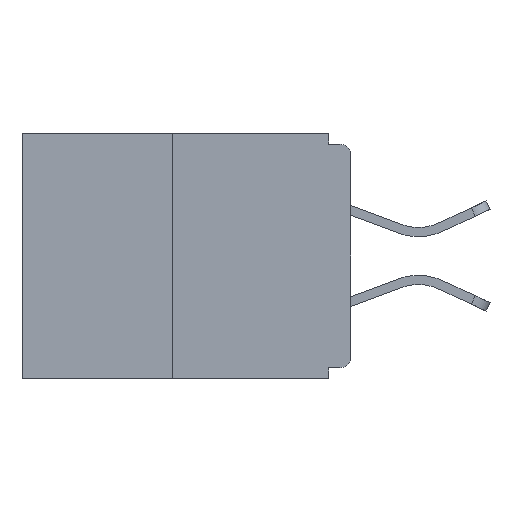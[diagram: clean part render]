
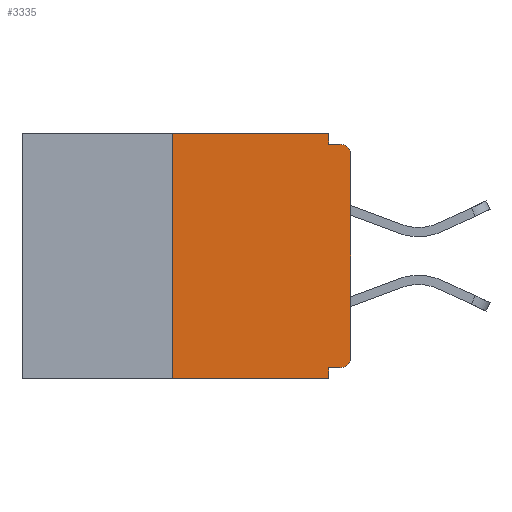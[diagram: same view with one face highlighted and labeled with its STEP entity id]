
A CAD part, left-side view. The second image highlights one B-rep face of the part: STEP entity #3335.
In plain terms, the highlighted planar face has unit normal (-1, 0, 0).
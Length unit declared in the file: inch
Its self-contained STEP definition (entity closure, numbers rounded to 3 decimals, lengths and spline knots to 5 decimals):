
#395 = EDGE_CURVE ( 'NONE', #3561, #10887, #11701, .T. ) ;
#424 = ORIENTED_EDGE ( 'NONE', *, *, #395, .F. ) ;
#631 = AXIS2_PLACEMENT_3D ( 'NONE', #7756, #4073, #10716 ) ;
#733 = AXIS2_PLACEMENT_3D ( 'NONE', #6651, #11321, #5610 ) ;
#974 = EDGE_CURVE ( 'NONE', #9422, #10626, #7133, .T. ) ;
#1036 = CARTESIAN_POINT ( 'NONE',  ( 0., 0.031, -0.015 ) ) ;
#1272 = LINE ( 'NONE', #4198, #9743 ) ;
#1452 = DIRECTION ( 'NONE',  ( 0., 0., 1. ) ) ;
#1589 = DIRECTION ( 'NONE',  ( -1., 0., 0. ) ) ;
#1690 = CARTESIAN_POINT ( 'NONE',  ( 0., 0.015, -0.313 ) ) ;
#2043 = DIRECTION ( 'NONE',  ( 0., -1., 0. ) ) ;
#2062 = ORIENTED_EDGE ( 'NONE', *, *, #2302, .F. ) ;
#2302 = EDGE_CURVE ( 'NONE', #11310, #5350, #6602, .T. ) ;
#2515 = CARTESIAN_POINT ( 'NONE',  ( 0., 0.015, -0.015 ) ) ;
#2636 = CARTESIAN_POINT ( 'NONE',  ( 0., 0.015, -0.328 ) ) ;
#2792 = VECTOR ( 'NONE', #6724, 39.37008 ) ;
#2806 = ORIENTED_EDGE ( 'NONE', *, *, #4476, .T. ) ;
#3335 = ADVANCED_FACE ( 'NONE', ( #8786 ), #8521, .F. ) ;
#3561 = VERTEX_POINT ( 'NONE', #5528 ) ;
#3802 = CARTESIAN_POINT ( 'NONE',  ( 0., 0., -0.03 ) ) ;
#3863 = CARTESIAN_POINT ( 'NONE',  ( 0., 0., -0.328 ) ) ;
#4073 = DIRECTION ( 'NONE',  ( -1., 0., 0. ) ) ;
#4198 = CARTESIAN_POINT ( 'NONE',  ( 0., 0.25, 0. ) ) ;
#4236 = VECTOR ( 'NONE', #1452, 39.37008 ) ;
#4357 = CARTESIAN_POINT ( 'NONE',  ( 0., 0.031, -0.343 ) ) ;
#4476 = EDGE_CURVE ( 'NONE', #5904, #5350, #11220, .T. ) ;
#4690 = LINE ( 'NONE', #7128, #4236 ) ;
#4773 = ORIENTED_EDGE ( 'NONE', *, *, #9515, .F. ) ;
#4829 = VECTOR ( 'NONE', #5130, 39.37008 ) ;
#4846 = CARTESIAN_POINT ( 'NONE',  ( 0., 0., -0.313 ) ) ;
#4853 = EDGE_CURVE ( 'NONE', #8885, #10826, #8806, .T. ) ;
#4958 = DIRECTION ( 'NONE',  ( 0., 0., 1. ) ) ;
#5130 = DIRECTION ( 'NONE',  ( 0., 0., -1. ) ) ;
#5167 = EDGE_CURVE ( 'NONE', #10887, #10626, #6867, .T. ) ;
#5242 = VECTOR ( 'NONE', #2043, 39.37008 ) ;
#5350 = VERTEX_POINT ( 'NONE', #4357 ) ;
#5528 = CARTESIAN_POINT ( 'NONE',  ( 0., 0.031, 0. ) ) ;
#5610 = DIRECTION ( 'NONE',  ( 0., 0., -1. ) ) ;
#5904 = VERTEX_POINT ( 'NONE', #11522 ) ;
#6077 = ORIENTED_EDGE ( 'NONE', *, *, #9986, .T. ) ;
#6602 = LINE ( 'NONE', #10877, #4829 ) ;
#6651 = CARTESIAN_POINT ( 'NONE',  ( 0., 0.46, 0. ) ) ;
#6724 = DIRECTION ( 'NONE',  ( 0., 0., -1. ) ) ;
#6867 = LINE ( 'NONE', #7733, #5242 ) ;
#7065 = EDGE_LOOP ( 'NONE', ( #8903, #10130, #2806, #2062, #4773, #9721, #6077, #9831, #12045, #424 ) ) ;
#7128 = CARTESIAN_POINT ( 'NONE',  ( 0., 0., 0. ) ) ;
#7133 = CIRCLE ( 'NONE', #631, 0.015 ) ;
#7208 = DIRECTION ( 'NONE',  ( 0., 0., -1. ) ) ;
#7671 = CARTESIAN_POINT ( 'NONE',  ( 0., 0.031, 0. ) ) ;
#7733 = CARTESIAN_POINT ( 'NONE',  ( 0., 0., -0.015 ) ) ;
#7756 = CARTESIAN_POINT ( 'NONE',  ( 0., 0.015, -0.03 ) ) ;
#7925 = VECTOR ( 'NONE', #12298, 39.37008 ) ;
#8292 = CARTESIAN_POINT ( 'NONE',  ( 0., 0.46, 0. ) ) ;
#8434 = DIRECTION ( 'NONE',  ( 0., 1., 0. ) ) ;
#8521 = PLANE ( 'NONE',  #733 ) ;
#8569 = EDGE_CURVE ( 'NONE', #9332, #3561, #10972, .T. ) ;
#8661 = DIRECTION ( 'NONE',  ( 0., -1., 0. ) ) ;
#8786 = FACE_OUTER_BOUND ( 'NONE', #7065, .T. ) ;
#8806 = CIRCLE ( 'NONE', #9650, 0.015 ) ;
#8885 = VERTEX_POINT ( 'NONE', #2636 ) ;
#8903 = ORIENTED_EDGE ( 'NONE', *, *, #8569, .F. ) ;
#9139 = CARTESIAN_POINT ( 'NONE',  ( 0., 0.031, -0.328 ) ) ;
#9315 = VECTOR ( 'NONE', #8661, 39.37008 ) ;
#9332 = VERTEX_POINT ( 'NONE', #11572 ) ;
#9422 = VERTEX_POINT ( 'NONE', #3802 ) ;
#9515 = EDGE_CURVE ( 'NONE', #8885, #11310, #10366, .T. ) ;
#9650 = AXIS2_PLACEMENT_3D ( 'NONE', #1690, #1589, #7208 ) ;
#9721 = ORIENTED_EDGE ( 'NONE', *, *, #4853, .T. ) ;
#9743 = VECTOR ( 'NONE', #4958, 39.37008 ) ;
#9823 = EDGE_CURVE ( 'NONE', #5904, #9332, #1272, .T. ) ;
#9831 = ORIENTED_EDGE ( 'NONE', *, *, #974, .T. ) ;
#9986 = EDGE_CURVE ( 'NONE', #10826, #9422, #4690, .T. ) ;
#10130 = ORIENTED_EDGE ( 'NONE', *, *, #9823, .F. ) ;
#10366 = LINE ( 'NONE', #3863, #10512 ) ;
#10512 = VECTOR ( 'NONE', #8434, 39.37008 ) ;
#10626 = VERTEX_POINT ( 'NONE', #2515 ) ;
#10716 = DIRECTION ( 'NONE',  ( 0., 0., -1. ) ) ;
#10826 = VERTEX_POINT ( 'NONE', #4846 ) ;
#10877 = CARTESIAN_POINT ( 'NONE',  ( 0., 0.031, -0.343 ) ) ;
#10887 = VERTEX_POINT ( 'NONE', #1036 ) ;
#10972 = LINE ( 'NONE', #8292, #9315 ) ;
#11220 = LINE ( 'NONE', #12266, #7925 ) ;
#11310 = VERTEX_POINT ( 'NONE', #9139 ) ;
#11321 = DIRECTION ( 'NONE',  ( 1., 0., 0. ) ) ;
#11522 = CARTESIAN_POINT ( 'NONE',  ( 0., 0.25, -0.343 ) ) ;
#11572 = CARTESIAN_POINT ( 'NONE',  ( 0., 0.25, 0. ) ) ;
#11701 = LINE ( 'NONE', #7671, #2792 ) ;
#12045 = ORIENTED_EDGE ( 'NONE', *, *, #5167, .F. ) ;
#12266 = CARTESIAN_POINT ( 'NONE',  ( 0., 0.46, -0.343 ) ) ;
#12298 = DIRECTION ( 'NONE',  ( 0., -1., 0. ) ) ;
